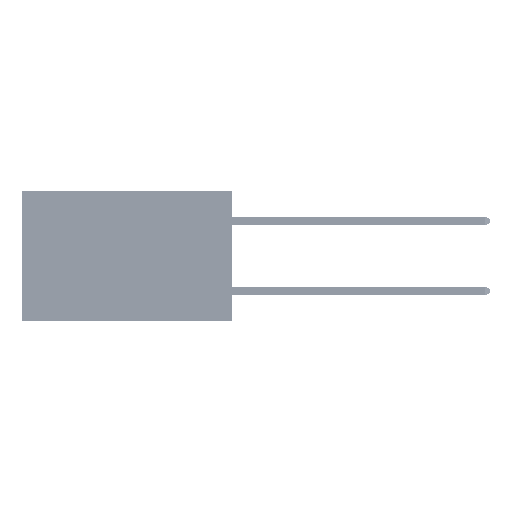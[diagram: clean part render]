
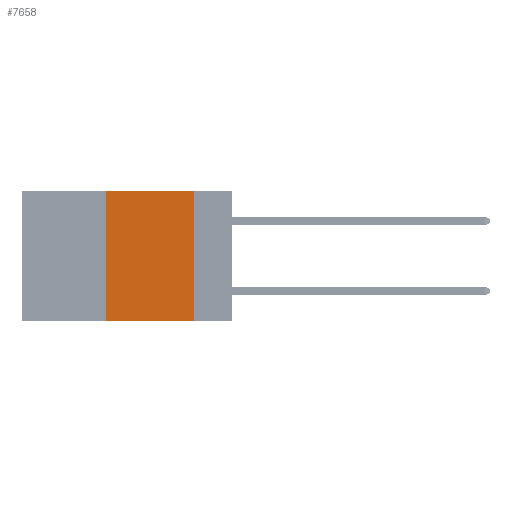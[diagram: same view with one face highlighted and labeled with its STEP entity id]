
A CAD part, left-side view. The second image highlights one B-rep face of the part: STEP entity #7658.
In plain terms, the highlighted planar face has unit normal (-1, 0, 0).
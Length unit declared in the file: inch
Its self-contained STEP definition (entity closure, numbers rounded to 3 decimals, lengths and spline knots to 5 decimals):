
#177 = LINE ( 'NONE', #11211, #19327 ) ;
#1152 = CARTESIAN_POINT ( 'NONE',  ( 0., 0.6, -0.37 ) ) ;
#3449 = CARTESIAN_POINT ( 'NONE',  ( 0., 0.11, -0.37 ) ) ;
#3602 = ORIENTED_EDGE ( 'NONE', *, *, #4885, .F. ) ;
#4302 = AXIS2_PLACEMENT_3D ( 'NONE', #49765, #9392, #37788 ) ;
#4885 = EDGE_CURVE ( 'NONE', #47827, #39056, #177, .T. ) ;
#5278 = DIRECTION ( 'NONE',  ( 0., -1., 0. ) ) ;
#5281 = PLANE ( 'NONE',  #4302 ) ;
#7502 = DIRECTION ( 'NONE',  ( 0., 0., -1. ) ) ;
#7658 = ADVANCED_FACE ( 'NONE', ( #13289 ), #5281, .F. ) ;
#9392 = DIRECTION ( 'NONE',  ( 1., 0., 0. ) ) ;
#9880 = EDGE_CURVE ( 'NONE', #39056, #12070, #36596, .T. ) ;
#11211 = CARTESIAN_POINT ( 'NONE',  ( 0., 0.36, 0. ) ) ;
#12070 = VERTEX_POINT ( 'NONE', #24166 ) ;
#13289 = FACE_OUTER_BOUND ( 'NONE', #48175, .T. ) ;
#13691 = ORIENTED_EDGE ( 'NONE', *, *, #9880, .F. ) ;
#14123 = EDGE_CURVE ( 'NONE', #12070, #18217, #42011, .T. ) ;
#15534 = VECTOR ( 'NONE', #5278, 39.37008 ) ;
#18217 = VERTEX_POINT ( 'NONE', #3449 ) ;
#19327 = VECTOR ( 'NONE', #43633, 39.37008 ) ;
#19431 = ORIENTED_EDGE ( 'NONE', *, *, #14123, .F. ) ;
#22585 = EDGE_CURVE ( 'NONE', #47827, #18217, #37130, .T. ) ;
#23272 = VECTOR ( 'NONE', #31570, 39.37008 ) ;
#24166 = CARTESIAN_POINT ( 'NONE',  ( 0., 0.11, 0. ) ) ;
#28918 = CARTESIAN_POINT ( 'NONE',  ( 0., 0.36, -0.37 ) ) ;
#31570 = DIRECTION ( 'NONE',  ( 0., -1., 0. ) ) ;
#34318 = ORIENTED_EDGE ( 'NONE', *, *, #22585, .T. ) ;
#35468 = CARTESIAN_POINT ( 'NONE',  ( 0., 0.6, 0. ) ) ;
#35906 = CARTESIAN_POINT ( 'NONE',  ( 0., 0.11, 0. ) ) ;
#36596 = LINE ( 'NONE', #35468, #23272 ) ;
#37130 = LINE ( 'NONE', #1152, #15534 ) ;
#37788 = DIRECTION ( 'NONE',  ( 0., 0., -1. ) ) ;
#38908 = CARTESIAN_POINT ( 'NONE',  ( 0., 0.36, 0. ) ) ;
#39056 = VERTEX_POINT ( 'NONE', #38908 ) ;
#42011 = LINE ( 'NONE', #35906, #51444 ) ;
#43633 = DIRECTION ( 'NONE',  ( 0., 0., 1. ) ) ;
#47827 = VERTEX_POINT ( 'NONE', #28918 ) ;
#48175 = EDGE_LOOP ( 'NONE', ( #19431, #13691, #3602, #34318 ) ) ;
#49765 = CARTESIAN_POINT ( 'NONE',  ( 0., 0.6, 0. ) ) ;
#51444 = VECTOR ( 'NONE', #7502, 39.37008 ) ;
